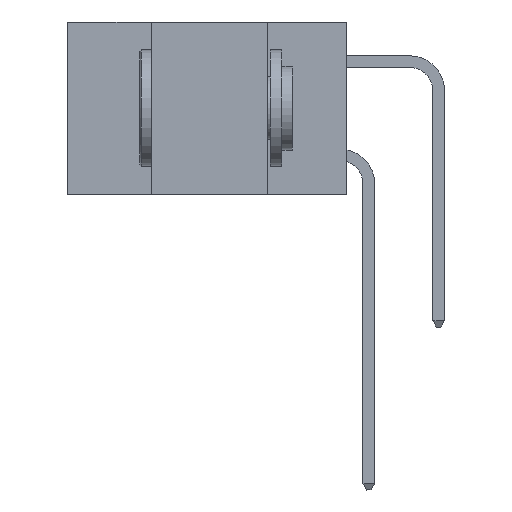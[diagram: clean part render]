
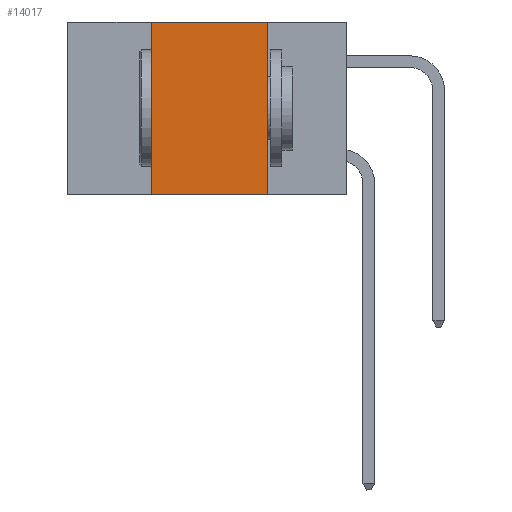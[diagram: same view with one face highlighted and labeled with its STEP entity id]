
A CAD part, left-side view. The second image highlights one B-rep face of the part: STEP entity #14017.
In plain terms, the highlighted planar face has unit normal (-1, 0, 0).
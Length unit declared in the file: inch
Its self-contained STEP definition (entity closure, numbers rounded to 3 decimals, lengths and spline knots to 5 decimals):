
#171 = EDGE_CURVE ( 'NONE', #13153, #5126, #11458, .T. ) ;
#1273 = PLANE ( 'NONE',  #9527 ) ;
#3370 = LINE ( 'NONE', #4502, #22770 ) ;
#3886 = ORIENTED_EDGE ( 'NONE', *, *, #171, .F. ) ;
#4502 = CARTESIAN_POINT ( 'NONE',  ( 0., 0.6, -0.37 ) ) ;
#4602 = VERTEX_POINT ( 'NONE', #9669 ) ;
#5126 = VERTEX_POINT ( 'NONE', #15226 ) ;
#5550 = VECTOR ( 'NONE', #21943, 39.37008 ) ;
#6267 = FACE_OUTER_BOUND ( 'NONE', #14170, .T. ) ;
#6338 = EDGE_CURVE ( 'NONE', #4602, #13153, #19259, .T. ) ;
#6893 = ORIENTED_EDGE ( 'NONE', *, *, #6338, .F. ) ;
#7439 = CARTESIAN_POINT ( 'NONE',  ( 0., 0.42, 0. ) ) ;
#7812 = CARTESIAN_POINT ( 'NONE',  ( 0., 0.42, 0. ) ) ;
#9527 = AXIS2_PLACEMENT_3D ( 'NONE', #14359, #12412, #19943 ) ;
#9669 = CARTESIAN_POINT ( 'NONE',  ( 0., 0.42, -0.37 ) ) ;
#10251 = DIRECTION ( 'NONE',  ( 0., -1., 0. ) ) ;
#10990 = CARTESIAN_POINT ( 'NONE',  ( 0., 0.17, 0. ) ) ;
#11458 = LINE ( 'NONE', #19875, #5550 ) ;
#12412 = DIRECTION ( 'NONE',  ( 1., 0., 0. ) ) ;
#13153 = VERTEX_POINT ( 'NONE', #7812 ) ;
#13901 = EDGE_CURVE ( 'NONE', #4602, #16716, #3370, .T. ) ;
#14017 = ADVANCED_FACE ( 'NONE', ( #6267 ), #1273, .F. ) ;
#14170 = EDGE_LOOP ( 'NONE', ( #21245, #3886, #6893, #22547 ) ) ;
#14359 = CARTESIAN_POINT ( 'NONE',  ( 0., 0.6, 0. ) ) ;
#15226 = CARTESIAN_POINT ( 'NONE',  ( 0., 0.17, 0. ) ) ;
#15974 = CARTESIAN_POINT ( 'NONE',  ( 0., 0.17, -0.37 ) ) ;
#16123 = EDGE_CURVE ( 'NONE', #5126, #16716, #21463, .T. ) ;
#16483 = VECTOR ( 'NONE', #21879, 39.37008 ) ;
#16716 = VERTEX_POINT ( 'NONE', #15974 ) ;
#18962 = VECTOR ( 'NONE', #22633, 39.37008 ) ;
#19259 = LINE ( 'NONE', #7439, #18962 ) ;
#19875 = CARTESIAN_POINT ( 'NONE',  ( 0., 0.6, 0. ) ) ;
#19943 = DIRECTION ( 'NONE',  ( 0., 0., -1. ) ) ;
#21245 = ORIENTED_EDGE ( 'NONE', *, *, #16123, .F. ) ;
#21463 = LINE ( 'NONE', #10990, #16483 ) ;
#21879 = DIRECTION ( 'NONE',  ( 0., 0., -1. ) ) ;
#21943 = DIRECTION ( 'NONE',  ( 0., -1., 0. ) ) ;
#22547 = ORIENTED_EDGE ( 'NONE', *, *, #13901, .T. ) ;
#22633 = DIRECTION ( 'NONE',  ( 0., 0., 1. ) ) ;
#22770 = VECTOR ( 'NONE', #10251, 39.37008 ) ;
